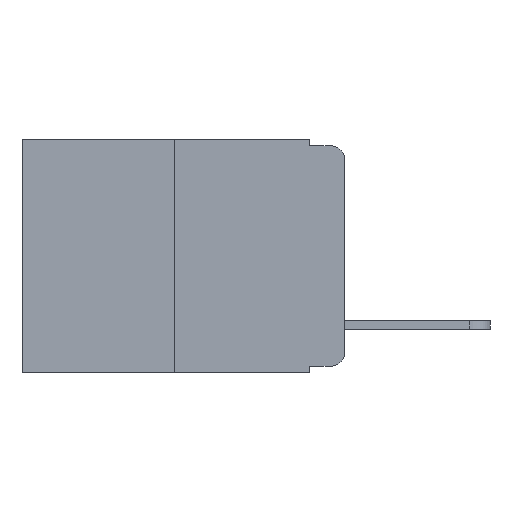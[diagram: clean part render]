
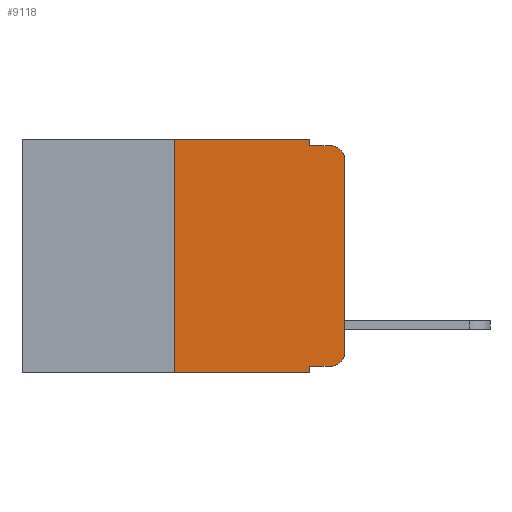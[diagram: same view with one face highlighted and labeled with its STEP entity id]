
A CAD part, left-side view. The second image highlights one B-rep face of the part: STEP entity #9118.
In plain terms, the highlighted planar face has unit normal (-1, 0, 0).
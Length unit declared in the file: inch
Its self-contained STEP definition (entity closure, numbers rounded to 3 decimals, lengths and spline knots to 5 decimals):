
#2 = VERTEX_POINT ( 'NONE', #7625 ) ;
#259 = DIRECTION ( 'NONE',  ( 0., -1., 0. ) ) ;
#426 = DIRECTION ( 'NONE',  ( 0., 0., -1. ) ) ;
#513 = CARTESIAN_POINT ( 'NONE',  ( 0., 0.051, -0.01 ) ) ;
#563 = VERTEX_POINT ( 'NONE', #8016 ) ;
#625 = VERTEX_POINT ( 'NONE', #6749 ) ;
#916 = CARTESIAN_POINT ( 'NONE',  ( 0., 0.051, 0. ) ) ;
#984 = EDGE_CURVE ( 'NONE', #1130, #2991, #4604, .T. ) ;
#1130 = VERTEX_POINT ( 'NONE', #4563 ) ;
#1237 = CARTESIAN_POINT ( 'NONE',  ( 0., 0.051, -0.333 ) ) ;
#1316 = PLANE ( 'NONE',  #4246 ) ;
#1383 = EDGE_CURVE ( 'NONE', #625, #2330, #8475, .T. ) ;
#1385 = EDGE_CURVE ( 'NONE', #2330, #2, #3637, .T. ) ;
#1431 = EDGE_CURVE ( 'NONE', #10022, #2, #8199, .T. ) ;
#1442 = EDGE_CURVE ( 'NONE', #8259, #10022, #2224, .T. ) ;
#1463 = LINE ( 'NONE', #1237, #6783 ) ;
#1469 = EDGE_CURVE ( 'NONE', #1130, #2930, #7349, .T. ) ;
#1501 = EDGE_CURVE ( 'NONE', #5359, #2991, #1863, .T. ) ;
#1530 = EDGE_CURVE ( 'NONE', #5359, #563, #1463, .T. ) ;
#1548 = EDGE_CURVE ( 'NONE', #563, #625, #8901, .T. ) ;
#1619 = DIRECTION ( 'NONE',  ( 0., 0., 1. ) ) ;
#1863 = LINE ( 'NONE', #2458, #9471 ) ;
#2074 = VECTOR ( 'NONE', #8674, 39.37008 ) ;
#2224 = LINE ( 'NONE', #916, #11802 ) ;
#2300 = DIRECTION ( 'NONE',  ( 0., 0., -1. ) ) ;
#2330 = VERTEX_POINT ( 'NONE', #6079 ) ;
#2409 = ORIENTED_EDGE ( 'NONE', *, *, #1383, .T. ) ;
#2420 = CARTESIAN_POINT ( 'NONE',  ( 0., 0.02, -0.03 ) ) ;
#2438 = ORIENTED_EDGE ( 'NONE', *, *, #984, .T. ) ;
#2458 = CARTESIAN_POINT ( 'NONE',  ( 0., 0.051, 0. ) ) ;
#2531 = ORIENTED_EDGE ( 'NONE', *, *, #1469, .F. ) ;
#2676 = DIRECTION ( 'NONE',  ( 0., 0., -1. ) ) ;
#2853 = DIRECTION ( 'NONE',  ( -1., 0., 0. ) ) ;
#2886 = ORIENTED_EDGE ( 'NONE', *, *, #1431, .F. ) ;
#2930 = VERTEX_POINT ( 'NONE', #3172 ) ;
#2940 = CARTESIAN_POINT ( 'NONE',  ( 0., 0.051, 0. ) ) ;
#2949 = ORIENTED_EDGE ( 'NONE', *, *, #1501, .F. ) ;
#2991 = VERTEX_POINT ( 'NONE', #4605 ) ;
#3172 = CARTESIAN_POINT ( 'NONE',  ( 0., 0.25, 0. ) ) ;
#3637 = CIRCLE ( 'NONE', #6429, 0.02 ) ;
#3731 = EDGE_CURVE ( 'NONE', #2930, #8259, #10555, .T. ) ;
#3888 = ORIENTED_EDGE ( 'NONE', *, *, #1530, .T. ) ;
#4007 = ORIENTED_EDGE ( 'NONE', *, *, #1548, .T. ) ;
#4124 = CARTESIAN_POINT ( 'NONE',  ( 0., 0.473, -0.343 ) ) ;
#4246 = AXIS2_PLACEMENT_3D ( 'NONE', #8726, #8653, #8646 ) ;
#4563 = CARTESIAN_POINT ( 'NONE',  ( 0., 0.25, -0.343 ) ) ;
#4604 = LINE ( 'NONE', #4124, #2074 ) ;
#4605 = CARTESIAN_POINT ( 'NONE',  ( 0., 0.051, -0.343 ) ) ;
#4653 = ORIENTED_EDGE ( 'NONE', *, *, #3731, .F. ) ;
#4689 = EDGE_LOOP ( 'NONE', ( #2409, #8132, #2886, #5715, #4653, #2531, #2438, #2949, #3888, #4007 ) ) ;
#5359 = VERTEX_POINT ( 'NONE', #11637 ) ;
#5715 = ORIENTED_EDGE ( 'NONE', *, *, #1442, .F. ) ;
#6079 = CARTESIAN_POINT ( 'NONE',  ( 0., 0., -0.03 ) ) ;
#6255 = CARTESIAN_POINT ( 'NONE',  ( 0., 0.051, -0.01 ) ) ;
#6429 = AXIS2_PLACEMENT_3D ( 'NONE', #2420, #2853, #2676 ) ;
#6749 = CARTESIAN_POINT ( 'NONE',  ( 0., 0., -0.313 ) ) ;
#6783 = VECTOR ( 'NONE', #6812, 39.37008 ) ;
#6812 = DIRECTION ( 'NONE',  ( 0., -1., 0. ) ) ;
#7349 = LINE ( 'NONE', #9531, #11565 ) ;
#7416 = DIRECTION ( 'NONE',  ( 0., 0., -1. ) ) ;
#7559 = DIRECTION ( 'NONE',  ( -1., 0., 0. ) ) ;
#7625 = CARTESIAN_POINT ( 'NONE',  ( 0., 0.02, -0.01 ) ) ;
#7647 = VECTOR ( 'NONE', #259, 39.37008 ) ;
#7858 = FACE_OUTER_BOUND ( 'NONE', #4689, .T. ) ;
#8016 = CARTESIAN_POINT ( 'NONE',  ( 0., 0.02, -0.333 ) ) ;
#8132 = ORIENTED_EDGE ( 'NONE', *, *, #1385, .T. ) ;
#8199 = LINE ( 'NONE', #513, #7647 ) ;
#8246 = VECTOR ( 'NONE', #12208, 39.37008 ) ;
#8259 = VERTEX_POINT ( 'NONE', #2940 ) ;
#8338 = CARTESIAN_POINT ( 'NONE',  ( 0., 0.02, -0.313 ) ) ;
#8342 = CARTESIAN_POINT ( 'NONE',  ( 0., 0.473, 0. ) ) ;
#8475 = LINE ( 'NONE', #10175, #10767 ) ;
#8646 = DIRECTION ( 'NONE',  ( 0., 0., -1. ) ) ;
#8653 = DIRECTION ( 'NONE',  ( 1., 0., 0. ) ) ;
#8674 = DIRECTION ( 'NONE',  ( 0., -1., 0. ) ) ;
#8726 = CARTESIAN_POINT ( 'NONE',  ( 0., 0.473, 0. ) ) ;
#8901 = CIRCLE ( 'NONE', #9803, 0.02 ) ;
#9118 = ADVANCED_FACE ( 'NONE', ( #7858 ), #1316, .F. ) ;
#9397 = DIRECTION ( 'NONE',  ( 0., 0., 1. ) ) ;
#9471 = VECTOR ( 'NONE', #2300, 39.37008 ) ;
#9531 = CARTESIAN_POINT ( 'NONE',  ( 0., 0.25, 0. ) ) ;
#9803 = AXIS2_PLACEMENT_3D ( 'NONE', #8338, #7559, #7416 ) ;
#10022 = VERTEX_POINT ( 'NONE', #6255 ) ;
#10175 = CARTESIAN_POINT ( 'NONE',  ( 0., 0., 0. ) ) ;
#10555 = LINE ( 'NONE', #8342, #8246 ) ;
#10767 = VECTOR ( 'NONE', #1619, 39.37008 ) ;
#11565 = VECTOR ( 'NONE', #9397, 39.37008 ) ;
#11637 = CARTESIAN_POINT ( 'NONE',  ( 0., 0.051, -0.333 ) ) ;
#11802 = VECTOR ( 'NONE', #426, 39.37008 ) ;
#12208 = DIRECTION ( 'NONE',  ( 0., -1., 0. ) ) ;
